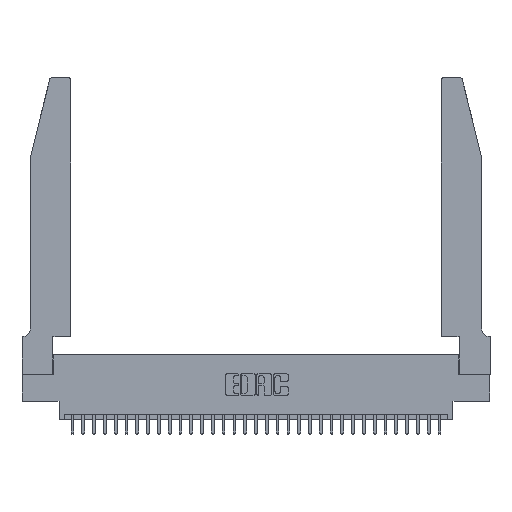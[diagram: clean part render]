
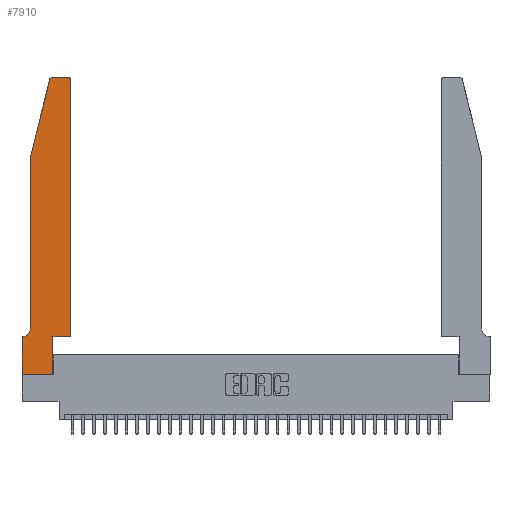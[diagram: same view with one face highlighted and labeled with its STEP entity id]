
A CAD part, top view. The second image highlights one B-rep face of the part: STEP entity #7910.
In plain terms, the highlighted planar face has unit normal (0, 0, 1).
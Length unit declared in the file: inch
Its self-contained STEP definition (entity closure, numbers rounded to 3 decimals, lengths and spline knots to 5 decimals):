
#190 = ORIENTED_EDGE ( 'NONE', *, *, #7428, .T. ) ;
#352 = VERTEX_POINT ( 'NONE', #16331 ) ;
#973 = CARTESIAN_POINT ( 'NONE',  ( 0.284, 2.72, 0.37 ) ) ;
#1207 = DIRECTION ( 'NONE',  ( -1., 0., 0. ) ) ;
#1314 = CARTESIAN_POINT ( 'NONE',  ( 0.0055, 0.42, 0.37 ) ) ;
#1417 = CARTESIAN_POINT ( 'NONE',  ( 0.0755, 0.35, 0.37 ) ) ;
#1587 = LINE ( 'NONE', #28598, #28207 ) ;
#2855 = CARTESIAN_POINT ( 'NONE',  ( 0., 0.35, 0.37 ) ) ;
#2934 = DIRECTION ( 'NONE',  ( 0., 1., 0. ) ) ;
#3155 = AXIS2_PLACEMENT_3D ( 'NONE', #2855, #28635, #13360 ) ;
#3415 = LINE ( 'NONE', #1417, #24000 ) ;
#3432 = LINE ( 'NONE', #15626, #18040 ) ;
#3579 = DIRECTION ( 'NONE',  ( 1., 0., 0. ) ) ;
#3666 = EDGE_CURVE ( 'NONE', #20071, #8146, #1587, .T. ) ;
#3922 = DIRECTION ( 'NONE',  ( -1., 0., 0. ) ) ;
#3943 = LINE ( 'NONE', #30111, #23722 ) ;
#3965 = CARTESIAN_POINT ( 'NONE',  ( 0.0755, 0.42, 0.37 ) ) ;
#4144 = CARTESIAN_POINT ( 'NONE',  ( 0.4205, 2.75, 0.37 ) ) ;
#4524 = VERTEX_POINT ( 'NONE', #4144 ) ;
#5006 = VERTEX_POINT ( 'NONE', #23971 ) ;
#5718 = CIRCLE ( 'NONE', #23557, 0.07 ) ;
#5762 = VERTEX_POINT ( 'NONE', #25083 ) ;
#6325 = CARTESIAN_POINT ( 'NONE',  ( 0., 0., 0.37 ) ) ;
#6911 = VECTOR ( 'NONE', #27429, 39.37008 ) ;
#6985 = EDGE_CURVE ( 'NONE', #8146, #352, #9958, .T. ) ;
#7114 = ORIENTED_EDGE ( 'NONE', *, *, #13313, .T. ) ;
#7231 = CARTESIAN_POINT ( 'NONE',  ( 0., 0., 0.37 ) ) ;
#7428 = EDGE_CURVE ( 'NONE', #7641, #20071, #16778, .T. ) ;
#7641 = VERTEX_POINT ( 'NONE', #7231 ) ;
#7657 = LINE ( 'NONE', #10246, #13761 ) ;
#7783 = ORIENTED_EDGE ( 'NONE', *, *, #18829, .T. ) ;
#7910 = ADVANCED_FACE ( 'NONE', ( #15149 ), #26087, .T. ) ;
#8146 = VERTEX_POINT ( 'NONE', #31959 ) ;
#9958 = LINE ( 'NONE', #14526, #29575 ) ;
#10246 = CARTESIAN_POINT ( 'NONE',  ( 0., 0., 0.37 ) ) ;
#10750 = VECTOR ( 'NONE', #29348, 39.37008 ) ;
#11902 = ORIENTED_EDGE ( 'NONE', *, *, #28431, .T. ) ;
#12854 = DIRECTION ( 'NONE',  ( 0., -1., 0. ) ) ;
#12915 = CARTESIAN_POINT ( 'NONE',  ( 0.0055, 0.35, 0.37 ) ) ;
#13147 = CARTESIAN_POINT ( 'NONE',  ( 0.284, 2.75, 0.37 ) ) ;
#13313 = EDGE_CURVE ( 'NONE', #25321, #16118, #5718, .T. ) ;
#13360 = DIRECTION ( 'NONE',  ( 1., 0., 0. ) ) ;
#13712 = VERTEX_POINT ( 'NONE', #13147 ) ;
#13761 = VECTOR ( 'NONE', #12854, 39.37008 ) ;
#13762 = CARTESIAN_POINT ( 'NONE',  ( 0.4505, 0.35, 0.37 ) ) ;
#14242 = VERTEX_POINT ( 'NONE', #20860 ) ;
#14392 = CARTESIAN_POINT ( 'NONE',  ( 0.4205, 2.72, 0.37 ) ) ;
#14526 = CARTESIAN_POINT ( 'NONE',  ( 0.4505, 0.35, 0.37 ) ) ;
#14594 = CARTESIAN_POINT ( 'NONE',  ( 0.0755, 2., 0.37 ) ) ;
#14712 = AXIS2_PLACEMENT_3D ( 'NONE', #973, #19095, #3579 ) ;
#14970 = ORIENTED_EDGE ( 'NONE', *, *, #21364, .T. ) ;
#15149 = FACE_OUTER_BOUND ( 'NONE', #29781, .T. ) ;
#15626 = CARTESIAN_POINT ( 'NONE',  ( 0.2605, 2.75, 0.37 ) ) ;
#16118 = VERTEX_POINT ( 'NONE', #12915 ) ;
#16331 = CARTESIAN_POINT ( 'NONE',  ( 0.4505, 0.35, 0.37 ) ) ;
#16341 = DIRECTION ( 'NONE',  ( 0., 1., 0. ) ) ;
#16778 = LINE ( 'NONE', #6325, #10750 ) ;
#16957 = DIRECTION ( 'NONE',  ( 1., 0., 0. ) ) ;
#17097 = DIRECTION ( 'NONE',  ( 1., 0., 0. ) ) ;
#17605 = ORIENTED_EDGE ( 'NONE', *, *, #30339, .T. ) ;
#18040 = VECTOR ( 'NONE', #23328, 39.37008 ) ;
#18829 = EDGE_CURVE ( 'NONE', #352, #5006, #30114, .T. ) ;
#19095 = DIRECTION ( 'NONE',  ( 0., 0., 1. ) ) ;
#19444 = DIRECTION ( 'NONE',  ( 0., 0., -1. ) ) ;
#19500 = EDGE_CURVE ( 'NONE', #13712, #25384, #24475, .T. ) ;
#19608 = EDGE_CURVE ( 'NONE', #5006, #4524, #22097, .T. ) ;
#19745 = EDGE_CURVE ( 'NONE', #25384, #14242, #3943, .T. ) ;
#20071 = VERTEX_POINT ( 'NONE', #28199 ) ;
#20860 = CARTESIAN_POINT ( 'NONE',  ( 0.0755, 2., 0.37 ) ) ;
#21364 = EDGE_CURVE ( 'NONE', #4524, #13712, #3432, .T. ) ;
#22097 = CIRCLE ( 'NONE', #30096, 0.03 ) ;
#23115 = ORIENTED_EDGE ( 'NONE', *, *, #19608, .T. ) ;
#23328 = DIRECTION ( 'NONE',  ( -1., 0., 0. ) ) ;
#23557 = AXIS2_PLACEMENT_3D ( 'NONE', #1314, #19444, #3922 ) ;
#23689 = ORIENTED_EDGE ( 'NONE', *, *, #3666, .T. ) ;
#23722 = VECTOR ( 'NONE', #32777, 39.37008 ) ;
#23971 = CARTESIAN_POINT ( 'NONE',  ( 0.4505, 2.72, 0.37 ) ) ;
#24000 = VECTOR ( 'NONE', #1207, 39.37008 ) ;
#24475 = CIRCLE ( 'NONE', #14712, 0.03 ) ;
#24637 = ORIENTED_EDGE ( 'NONE', *, *, #6985, .T. ) ;
#25083 = CARTESIAN_POINT ( 'NONE',  ( 0., 0.35, 0.37 ) ) ;
#25321 = VERTEX_POINT ( 'NONE', #3965 ) ;
#25384 = VERTEX_POINT ( 'NONE', #29846 ) ;
#26087 = PLANE ( 'NONE',  #3155 ) ;
#27299 = ORIENTED_EDGE ( 'NONE', *, *, #19745, .T. ) ;
#27412 = LINE ( 'NONE', #14594, #6911 ) ;
#27429 = DIRECTION ( 'NONE',  ( 0., -1., 0. ) ) ;
#28199 = CARTESIAN_POINT ( 'NONE',  ( 0.2865, 0., 0.37 ) ) ;
#28207 = VECTOR ( 'NONE', #2934, 39.37008 ) ;
#28307 = ORIENTED_EDGE ( 'NONE', *, *, #31196, .T. ) ;
#28431 = EDGE_CURVE ( 'NONE', #16118, #5762, #3415, .T. ) ;
#28598 = CARTESIAN_POINT ( 'NONE',  ( 0.2865, 0.35, 0.37 ) ) ;
#28621 = ORIENTED_EDGE ( 'NONE', *, *, #19500, .T. ) ;
#28635 = DIRECTION ( 'NONE',  ( 0., 0., 1. ) ) ;
#29319 = VECTOR ( 'NONE', #16341, 39.37008 ) ;
#29348 = DIRECTION ( 'NONE',  ( 1., 0., 0. ) ) ;
#29575 = VECTOR ( 'NONE', #17097, 39.37008 ) ;
#29781 = EDGE_LOOP ( 'NONE', ( #14970, #28621, #27299, #17605, #7114, #11902, #28307, #190, #23689, #24637, #7783, #23115 ) ) ;
#29846 = CARTESIAN_POINT ( 'NONE',  ( 0.25487, 2.72718, 0.37 ) ) ;
#30096 = AXIS2_PLACEMENT_3D ( 'NONE', #14392, #32218, #16957 ) ;
#30111 = CARTESIAN_POINT ( 'NONE',  ( 0.0755, 2., 0.37 ) ) ;
#30114 = LINE ( 'NONE', #13762, #29319 ) ;
#30339 = EDGE_CURVE ( 'NONE', #14242, #25321, #27412, .T. ) ;
#31196 = EDGE_CURVE ( 'NONE', #5762, #7641, #7657, .T. ) ;
#31959 = CARTESIAN_POINT ( 'NONE',  ( 0.2865, 0.35, 0.37 ) ) ;
#32218 = DIRECTION ( 'NONE',  ( 0., 0., 1. ) ) ;
#32777 = DIRECTION ( 'NONE',  ( -0.239, -0.971, 0. ) ) ;
